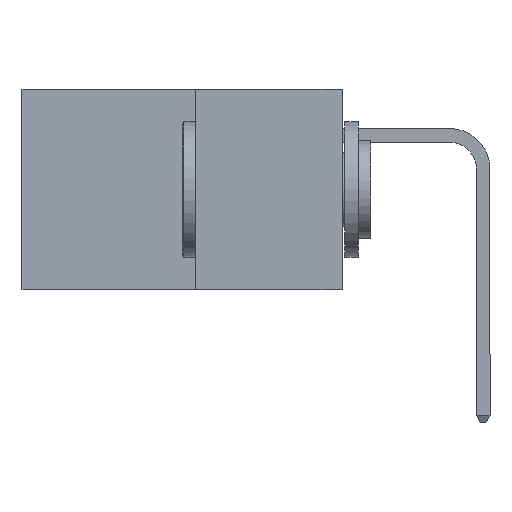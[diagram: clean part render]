
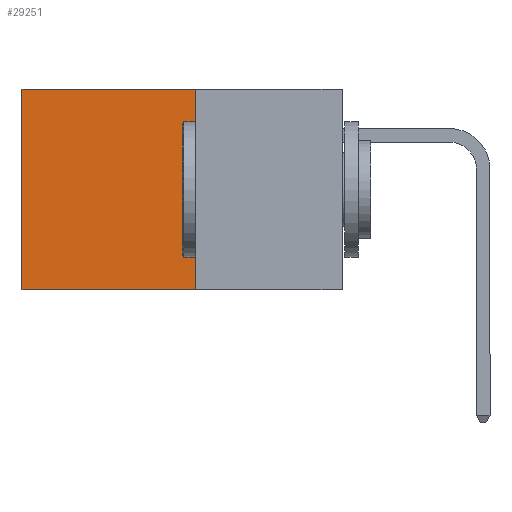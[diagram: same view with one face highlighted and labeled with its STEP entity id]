
A CAD part, left-side view. The second image highlights one B-rep face of the part: STEP entity #29251.
In plain terms, the highlighted planar face has unit normal (-1, 0, 0).
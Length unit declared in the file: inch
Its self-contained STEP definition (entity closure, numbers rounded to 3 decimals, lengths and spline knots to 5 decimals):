
#283 = VERTEX_POINT ( 'NONE', #21222 ) ;
#537 = PLANE ( 'NONE',  #11448 ) ;
#631 = DIRECTION ( 'NONE',  ( 1., 0., 0. ) ) ;
#1193 = ORIENTED_EDGE ( 'NONE', *, *, #4768, .F. ) ;
#2298 = CARTESIAN_POINT ( 'NONE',  ( 0.277, 0.59, 0. ) ) ;
#2340 = DIRECTION ( 'NONE',  ( 0., 0., -1. ) ) ;
#4327 = ORIENTED_EDGE ( 'NONE', *, *, #11796, .T. ) ;
#4768 = EDGE_CURVE ( 'NONE', #27549, #283, #28384, .T. ) ;
#6278 = FACE_OUTER_BOUND ( 'NONE', #10922, .T. ) ;
#8992 = CARTESIAN_POINT ( 'NONE',  ( 0.277, 0.59, -0.37 ) ) ;
#9177 = EDGE_CURVE ( 'NONE', #16737, #27097, #10487, .T. ) ;
#10163 = VECTOR ( 'NONE', #16532, 39.37008 ) ;
#10487 = LINE ( 'NONE', #24148, #28012 ) ;
#10578 = EDGE_CURVE ( 'NONE', #16737, #27549, #14339, .T. ) ;
#10922 = EDGE_LOOP ( 'NONE', ( #4327, #1193, #11817, #17277 ) ) ;
#11448 = AXIS2_PLACEMENT_3D ( 'NONE', #14389, #631, #16699 ) ;
#11796 = EDGE_CURVE ( 'NONE', #27097, #283, #22529, .T. ) ;
#11817 = ORIENTED_EDGE ( 'NONE', *, *, #10578, .F. ) ;
#13760 = CARTESIAN_POINT ( 'NONE',  ( 0.277, 0.27, -0.37 ) ) ;
#14339 = LINE ( 'NONE', #13760, #19779 ) ;
#14389 = CARTESIAN_POINT ( 'NONE',  ( 0.277, 0.27, -0.37 ) ) ;
#14637 = CARTESIAN_POINT ( 'NONE',  ( 0.277, 0.27, 0. ) ) ;
#15022 = DIRECTION ( 'NONE',  ( 0., 1., 0. ) ) ;
#16500 = CARTESIAN_POINT ( 'NONE',  ( 0.277, 0.27, -0.37 ) ) ;
#16532 = DIRECTION ( 'NONE',  ( 0., 1., 0. ) ) ;
#16699 = DIRECTION ( 'NONE',  ( 0., 0., -1. ) ) ;
#16737 = VERTEX_POINT ( 'NONE', #14637 ) ;
#17277 = ORIENTED_EDGE ( 'NONE', *, *, #9177, .T. ) ;
#19779 = VECTOR ( 'NONE', #2340, 39.37008 ) ;
#21222 = CARTESIAN_POINT ( 'NONE',  ( 0.277, 0.59, -0.37 ) ) ;
#22529 = LINE ( 'NONE', #8992, #27849 ) ;
#24148 = CARTESIAN_POINT ( 'NONE',  ( 0.277, 0.27, 0. ) ) ;
#26602 = CARTESIAN_POINT ( 'NONE',  ( 0.277, 0.27, -0.37 ) ) ;
#27097 = VERTEX_POINT ( 'NONE', #2298 ) ;
#27549 = VERTEX_POINT ( 'NONE', #26602 ) ;
#27849 = VECTOR ( 'NONE', #29444, 39.37008 ) ;
#28012 = VECTOR ( 'NONE', #15022, 39.37008 ) ;
#28384 = LINE ( 'NONE', #16500, #10163 ) ;
#29251 = ADVANCED_FACE ( 'NONE', ( #6278 ), #537, .F. ) ;
#29444 = DIRECTION ( 'NONE',  ( 0., 0., -1. ) ) ;
